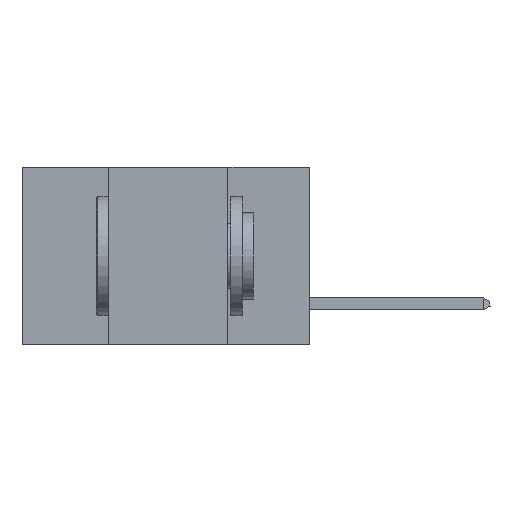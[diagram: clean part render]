
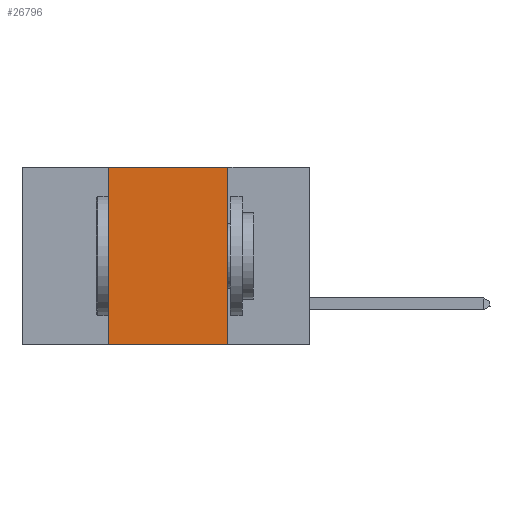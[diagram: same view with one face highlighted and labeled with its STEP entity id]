
A CAD part, left-side view. The second image highlights one B-rep face of the part: STEP entity #26796.
In plain terms, the highlighted planar face has unit normal (-1, 0, 0).
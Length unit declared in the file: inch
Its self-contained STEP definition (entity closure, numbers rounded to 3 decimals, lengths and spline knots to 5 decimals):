
#656 = ORIENTED_EDGE ( 'NONE', *, *, #16921, .F. ) ;
#1130 = DIRECTION ( 'NONE',  ( 0., 0., -1. ) ) ;
#3474 = FACE_OUTER_BOUND ( 'NONE', #27613, .T. ) ;
#5719 = DIRECTION ( 'NONE',  ( 0., 0., -1. ) ) ;
#7387 = CARTESIAN_POINT ( 'NONE',  ( 0., 0.42, 0. ) ) ;
#9402 = VECTOR ( 'NONE', #5719, 39.37008 ) ;
#9403 = CARTESIAN_POINT ( 'NONE',  ( 0., 0.6, 0. ) ) ;
#11989 = ORIENTED_EDGE ( 'NONE', *, *, #12974, .F. ) ;
#12974 = EDGE_CURVE ( 'NONE', #15632, #33845, #46175, .T. ) ;
#13657 = LINE ( 'NONE', #30256, #22885 ) ;
#14947 = DIRECTION ( 'NONE',  ( 0., -1., 0. ) ) ;
#15617 = CARTESIAN_POINT ( 'NONE',  ( 0., 0.42, -0.37 ) ) ;
#15632 = VERTEX_POINT ( 'NONE', #15617 ) ;
#16921 = EDGE_CURVE ( 'NONE', #35064, #25852, #48261, .T. ) ;
#17802 = EDGE_CURVE ( 'NONE', #15632, #25852, #13657, .T. ) ;
#19077 = LINE ( 'NONE', #34897, #28075 ) ;
#21651 = CARTESIAN_POINT ( 'NONE',  ( 0., 0.17, 0. ) ) ;
#22108 = AXIS2_PLACEMENT_3D ( 'NONE', #9403, #32231, #1130 ) ;
#22885 = VECTOR ( 'NONE', #14947, 39.37008 ) ;
#24712 = PLANE ( 'NONE',  #22108 ) ;
#24795 = VECTOR ( 'NONE', #38370, 39.37008 ) ;
#25852 = VERTEX_POINT ( 'NONE', #28769 ) ;
#25932 = CARTESIAN_POINT ( 'NONE',  ( 0., 0.17, 0. ) ) ;
#26796 = ADVANCED_FACE ( 'NONE', ( #3474 ), #24712, .F. ) ;
#27369 = DIRECTION ( 'NONE',  ( 0., -1., 0. ) ) ;
#27613 = EDGE_LOOP ( 'NONE', ( #656, #39673, #11989, #28857 ) ) ;
#28075 = VECTOR ( 'NONE', #27369, 39.37008 ) ;
#28769 = CARTESIAN_POINT ( 'NONE',  ( 0., 0.17, -0.37 ) ) ;
#28857 = ORIENTED_EDGE ( 'NONE', *, *, #17802, .T. ) ;
#30256 = CARTESIAN_POINT ( 'NONE',  ( 0., 0.6, -0.37 ) ) ;
#31159 = EDGE_CURVE ( 'NONE', #33845, #35064, #19077, .T. ) ;
#32144 = CARTESIAN_POINT ( 'NONE',  ( 0., 0.42, 0. ) ) ;
#32231 = DIRECTION ( 'NONE',  ( 1., 0., 0. ) ) ;
#33845 = VERTEX_POINT ( 'NONE', #32144 ) ;
#34897 = CARTESIAN_POINT ( 'NONE',  ( 0., 0.6, 0. ) ) ;
#35064 = VERTEX_POINT ( 'NONE', #25932 ) ;
#38370 = DIRECTION ( 'NONE',  ( 0., 0., 1. ) ) ;
#39673 = ORIENTED_EDGE ( 'NONE', *, *, #31159, .F. ) ;
#46175 = LINE ( 'NONE', #7387, #24795 ) ;
#48261 = LINE ( 'NONE', #21651, #9402 ) ;
